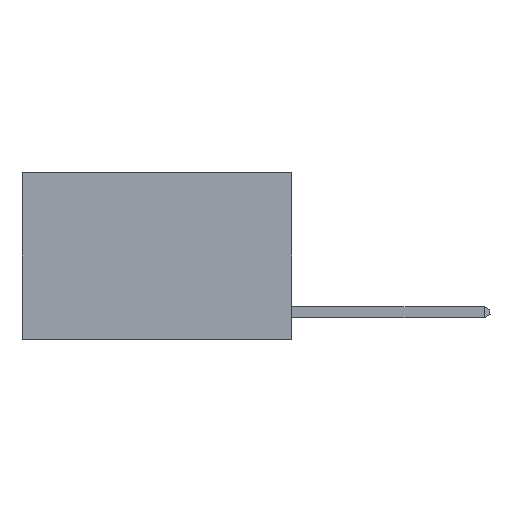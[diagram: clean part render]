
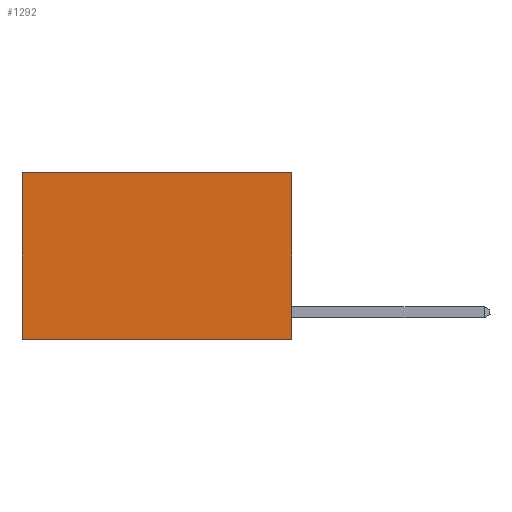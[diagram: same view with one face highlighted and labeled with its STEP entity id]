
A CAD part, left-side view. The second image highlights one B-rep face of the part: STEP entity #1292.
In plain terms, the highlighted planar face has unit normal (-1, 0, 0).
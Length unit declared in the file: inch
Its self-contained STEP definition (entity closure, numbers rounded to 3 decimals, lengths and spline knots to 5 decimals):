
#76 = CARTESIAN_POINT ( 'NONE',  ( 0.2625, 0., -0.37 ) ) ;
#460 = ORIENTED_EDGE ( 'NONE', *, *, #9453, .F. ) ;
#1080 = DIRECTION ( 'NONE',  ( 0., 1., 0. ) ) ;
#1292 = ADVANCED_FACE ( 'NONE', ( #7587 ), #4378, .F. ) ;
#1352 = CARTESIAN_POINT ( 'NONE',  ( 0.2625, 0., -0.37 ) ) ;
#1848 = EDGE_CURVE ( 'NONE', #10624, #12583, #2395, .T. ) ;
#1869 = VERTEX_POINT ( 'NONE', #11271 ) ;
#1925 = EDGE_LOOP ( 'NONE', ( #10268, #8248, #460, #11656 ) ) ;
#2147 = VERTEX_POINT ( 'NONE', #6361 ) ;
#2185 = VECTOR ( 'NONE', #1080, 39.37008 ) ;
#2395 = LINE ( 'NONE', #76, #2735 ) ;
#2735 = VECTOR ( 'NONE', #7218, 39.37008 ) ;
#3915 = EDGE_CURVE ( 'NONE', #2147, #12583, #5419, .T. ) ;
#4378 = PLANE ( 'NONE',  #11004 ) ;
#4634 = LINE ( 'NONE', #5206, #2185 ) ;
#5045 = VECTOR ( 'NONE', #7269, 39.37008 ) ;
#5206 = CARTESIAN_POINT ( 'NONE',  ( 0.2625, 0., 0. ) ) ;
#5232 = CARTESIAN_POINT ( 'NONE',  ( 0.2625, 0., 0. ) ) ;
#5295 = CARTESIAN_POINT ( 'NONE',  ( 0.2625, 0., 0. ) ) ;
#5419 = LINE ( 'NONE', #6340, #10506 ) ;
#5899 = DIRECTION ( 'NONE',  ( 1., 0., 0. ) ) ;
#5946 = CARTESIAN_POINT ( 'NONE',  ( 0.2625, 0.6, -0.37 ) ) ;
#6340 = CARTESIAN_POINT ( 'NONE',  ( 0.2625, 0.6, 0. ) ) ;
#6361 = CARTESIAN_POINT ( 'NONE',  ( 0.2625, 0.6, 0. ) ) ;
#7218 = DIRECTION ( 'NONE',  ( 0., 1., 0. ) ) ;
#7269 = DIRECTION ( 'NONE',  ( 0., 0., -1. ) ) ;
#7374 = DIRECTION ( 'NONE',  ( 0., 0., -1. ) ) ;
#7451 = EDGE_CURVE ( 'NONE', #1869, #2147, #4634, .T. ) ;
#7491 = LINE ( 'NONE', #5232, #5045 ) ;
#7587 = FACE_OUTER_BOUND ( 'NONE', #1925, .T. ) ;
#8248 = ORIENTED_EDGE ( 'NONE', *, *, #1848, .F. ) ;
#9453 = EDGE_CURVE ( 'NONE', #1869, #10624, #7491, .T. ) ;
#10268 = ORIENTED_EDGE ( 'NONE', *, *, #3915, .T. ) ;
#10506 = VECTOR ( 'NONE', #7374, 39.37008 ) ;
#10511 = DIRECTION ( 'NONE',  ( 0., 0., -1. ) ) ;
#10624 = VERTEX_POINT ( 'NONE', #1352 ) ;
#11004 = AXIS2_PLACEMENT_3D ( 'NONE', #5295, #5899, #10511 ) ;
#11271 = CARTESIAN_POINT ( 'NONE',  ( 0.2625, 0., 0. ) ) ;
#11656 = ORIENTED_EDGE ( 'NONE', *, *, #7451, .T. ) ;
#12583 = VERTEX_POINT ( 'NONE', #5946 ) ;
